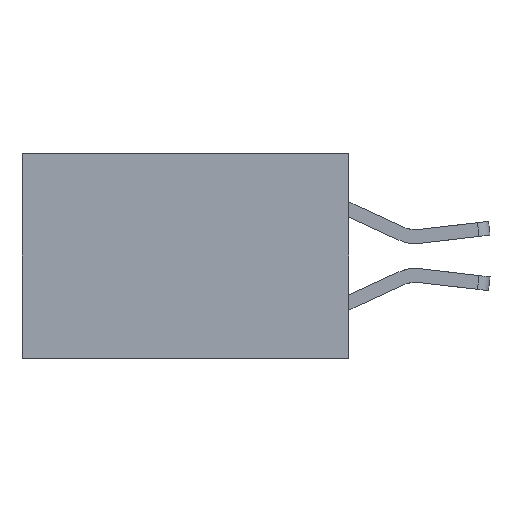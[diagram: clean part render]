
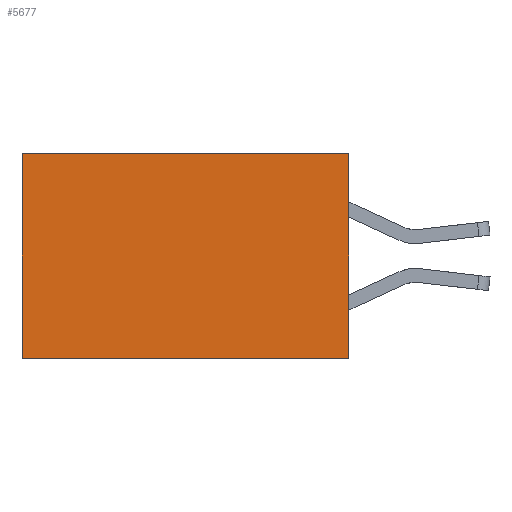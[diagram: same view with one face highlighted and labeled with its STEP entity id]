
A CAD part, left-side view. The second image highlights one B-rep face of the part: STEP entity #5677.
In plain terms, the highlighted planar face has unit normal (-1, 0, 0).
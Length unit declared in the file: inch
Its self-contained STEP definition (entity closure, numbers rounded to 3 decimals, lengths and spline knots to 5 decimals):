
#26 = CARTESIAN_POINT ( 'NONE',  ( 0.277, 0., 0. ) ) ;
#134 = DIRECTION ( 'NONE',  ( 0., 0., -1. ) ) ;
#655 = VECTOR ( 'NONE', #7247, 39.37008 ) ;
#803 = FACE_OUTER_BOUND ( 'NONE', #7095, .T. ) ;
#1286 = LINE ( 'NONE', #2311, #6326 ) ;
#1581 = ORIENTED_EDGE ( 'NONE', *, *, #3718, .T. ) ;
#1607 = ORIENTED_EDGE ( 'NONE', *, *, #1736, .T. ) ;
#1658 = ORIENTED_EDGE ( 'NONE', *, *, #3636, .F. ) ;
#1675 = ORIENTED_EDGE ( 'NONE', *, *, #8329, .F. ) ;
#1736 = EDGE_CURVE ( 'NONE', #1986, #3060, #4015, .T. ) ;
#1771 = CARTESIAN_POINT ( 'NONE',  ( 0.277, 0.59, 0. ) ) ;
#1986 = VERTEX_POINT ( 'NONE', #1771 ) ;
#2311 = CARTESIAN_POINT ( 'NONE',  ( 0.277, 0., 0. ) ) ;
#2336 = DIRECTION ( 'NONE',  ( 0., 1., 0. ) ) ;
#2934 = VERTEX_POINT ( 'NONE', #8128 ) ;
#3060 = VERTEX_POINT ( 'NONE', #6850 ) ;
#3233 = DIRECTION ( 'NONE',  ( 0., 0., -1. ) ) ;
#3361 = VECTOR ( 'NONE', #3233, 39.37008 ) ;
#3436 = CARTESIAN_POINT ( 'NONE',  ( 0.277, 0., -0.37 ) ) ;
#3531 = DIRECTION ( 'NONE',  ( 0., 0., -1. ) ) ;
#3537 = DIRECTION ( 'NONE',  ( 1., 0., 0. ) ) ;
#3552 = PLANE ( 'NONE',  #7209 ) ;
#3636 = EDGE_CURVE ( 'NONE', #7855, #2934, #6908, .T. ) ;
#3718 = EDGE_CURVE ( 'NONE', #7855, #1986, #1286, .T. ) ;
#3922 = CARTESIAN_POINT ( 'NONE',  ( 0.277, 0., -0.37 ) ) ;
#4015 = LINE ( 'NONE', #4768, #7525 ) ;
#4768 = CARTESIAN_POINT ( 'NONE',  ( 0.277, 0.59, -0.37 ) ) ;
#5677 = ADVANCED_FACE ( 'NONE', ( #803 ), #3552, .F. ) ;
#6326 = VECTOR ( 'NONE', #2336, 39.37008 ) ;
#6850 = CARTESIAN_POINT ( 'NONE',  ( 0.277, 0.59, -0.37 ) ) ;
#6908 = LINE ( 'NONE', #3436, #3361 ) ;
#7095 = EDGE_LOOP ( 'NONE', ( #1607, #1675, #1658, #1581 ) ) ;
#7209 = AXIS2_PLACEMENT_3D ( 'NONE', #3922, #3537, #3531 ) ;
#7232 = LINE ( 'NONE', #8610, #655 ) ;
#7247 = DIRECTION ( 'NONE',  ( 0., 1., 0. ) ) ;
#7525 = VECTOR ( 'NONE', #134, 39.37008 ) ;
#7855 = VERTEX_POINT ( 'NONE', #26 ) ;
#8128 = CARTESIAN_POINT ( 'NONE',  ( 0.277, 0., -0.37 ) ) ;
#8329 = EDGE_CURVE ( 'NONE', #2934, #3060, #7232, .T. ) ;
#8610 = CARTESIAN_POINT ( 'NONE',  ( 0.277, 0., -0.37 ) ) ;
